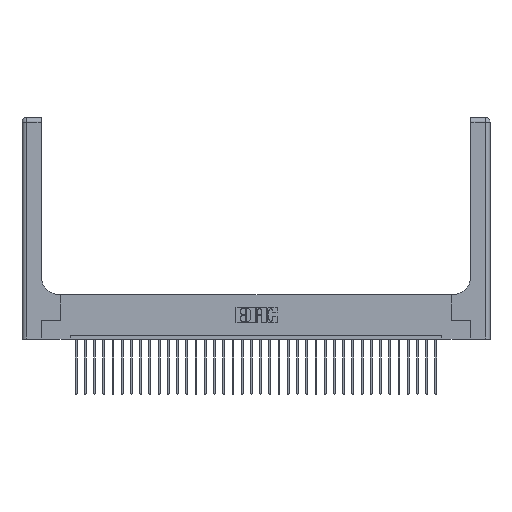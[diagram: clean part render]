
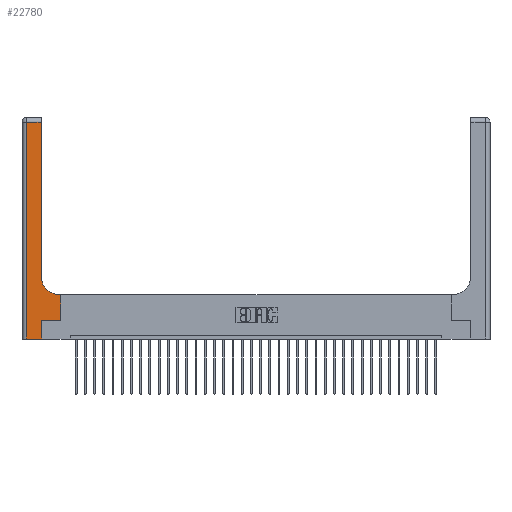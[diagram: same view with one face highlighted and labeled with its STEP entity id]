
A CAD part, top view. The second image highlights one B-rep face of the part: STEP entity #22780.
In plain terms, the highlighted planar face has unit normal (0, 0, 1).
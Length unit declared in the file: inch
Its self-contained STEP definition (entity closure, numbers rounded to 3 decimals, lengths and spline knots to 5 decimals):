
#1024 = CARTESIAN_POINT ( 'NONE',  ( 0.26, 2.94, 0.37 ) ) ;
#1397 = CARTESIAN_POINT ( 'NONE',  ( 0.26, 3., 0.37 ) ) ;
#1685 = CARTESIAN_POINT ( 'NONE',  ( 0., 3., 0.37 ) ) ;
#1891 = DIRECTION ( 'NONE',  ( 0., 0., -1. ) ) ;
#1976 = ORIENTED_EDGE ( 'NONE', *, *, #28139, .T. ) ;
#3897 = DIRECTION ( 'NONE',  ( 0., 1., 0. ) ) ;
#4067 = EDGE_CURVE ( 'NONE', #28895, #26135, #25489, .T. ) ;
#4307 = CARTESIAN_POINT ( 'NONE',  ( 0.06, 3., 0.37 ) ) ;
#4350 = CARTESIAN_POINT ( 'NONE',  ( 0.528, 0.25, 0.37 ) ) ;
#4663 = EDGE_CURVE ( 'NONE', #26135, #20665, #19609, .T. ) ;
#5077 = ORIENTED_EDGE ( 'NONE', *, *, #6929, .T. ) ;
#5150 = VECTOR ( 'NONE', #18084, 39.37008 ) ;
#6020 = ORIENTED_EDGE ( 'NONE', *, *, #16558, .T. ) ;
#6377 = VERTEX_POINT ( 'NONE', #14518 ) ;
#6764 = VECTOR ( 'NONE', #26221, 39.37008 ) ;
#6796 = EDGE_CURVE ( 'NONE', #28186, #12168, #22173, .T. ) ;
#6875 = LINE ( 'NONE', #29794, #18598 ) ;
#6929 = EDGE_CURVE ( 'NONE', #6377, #28895, #21804, .T. ) ;
#8192 = CARTESIAN_POINT ( 'NONE',  ( 0.51, 0.85, 0.37 ) ) ;
#8345 = VERTEX_POINT ( 'NONE', #26158 ) ;
#8560 = EDGE_CURVE ( 'NONE', #29387, #16786, #12880, .T. ) ;
#9217 = ORIENTED_EDGE ( 'NONE', *, *, #4663, .T. ) ;
#9361 = VECTOR ( 'NONE', #21177, 39.37008 ) ;
#9370 = CARTESIAN_POINT ( 'NONE',  ( 0.06, 0., 0.37 ) ) ;
#11215 = CARTESIAN_POINT ( 'NONE',  ( 0.528, 0.6, 0.37 ) ) ;
#11298 = DIRECTION ( 'NONE',  ( 0., -1., 0. ) ) ;
#11910 = FACE_OUTER_BOUND ( 'NONE', #14906, .T. ) ;
#12168 = VERTEX_POINT ( 'NONE', #1024 ) ;
#12880 = LINE ( 'NONE', #4307, #27166 ) ;
#13280 = ORIENTED_EDGE ( 'NONE', *, *, #8560, .T. ) ;
#13945 = CIRCLE ( 'NONE', #25752, 0.25 ) ;
#14185 = DIRECTION ( 'NONE',  ( -1., 0., 0. ) ) ;
#14518 = CARTESIAN_POINT ( 'NONE',  ( 0.265, 0.25, 0.37 ) ) ;
#14860 = ORIENTED_EDGE ( 'NONE', *, *, #6796, .T. ) ;
#14906 = EDGE_LOOP ( 'NONE', ( #14860, #6020, #13280, #19827, #1976, #5077, #29991, #9217, #23270 ) ) ;
#15052 = DIRECTION ( 'NONE',  ( 1., 0., 0. ) ) ;
#15379 = AXIS2_PLACEMENT_3D ( 'NONE', #1685, #1891, #22839 ) ;
#15448 = DIRECTION ( 'NONE',  ( 0., 0., -1. ) ) ;
#15474 = CARTESIAN_POINT ( 'NONE',  ( 0.26, 0.85, 0.37 ) ) ;
#15578 = PLANE ( 'NONE',  #15379 ) ;
#15915 = VECTOR ( 'NONE', #14185, 39.37008 ) ;
#16093 = CARTESIAN_POINT ( 'NONE',  ( 0., 0., 0.37 ) ) ;
#16178 = CARTESIAN_POINT ( 'NONE',  ( 0.528, 0.25, 0.37 ) ) ;
#16558 = EDGE_CURVE ( 'NONE', #12168, #29387, #22740, .T. ) ;
#16786 = VERTEX_POINT ( 'NONE', #9370 ) ;
#18084 = DIRECTION ( 'NONE',  ( -1., 0., 0. ) ) ;
#18189 = CARTESIAN_POINT ( 'NONE',  ( 0.51, 0.6, 0.37 ) ) ;
#18524 = DIRECTION ( 'NONE',  ( 0., 1., 0. ) ) ;
#18598 = VECTOR ( 'NONE', #3897, 39.37008 ) ;
#18666 = EDGE_CURVE ( 'NONE', #20665, #28186, #13945, .T. ) ;
#19609 = LINE ( 'NONE', #27932, #15915 ) ;
#19827 = ORIENTED_EDGE ( 'NONE', *, *, #22883, .T. ) ;
#20665 = VERTEX_POINT ( 'NONE', #18189 ) ;
#21053 = VECTOR ( 'NONE', #27157, 39.37008 ) ;
#21177 = DIRECTION ( 'NONE',  ( 1., 0., 0. ) ) ;
#21280 = CARTESIAN_POINT ( 'NONE',  ( 0.265, 0.25, 0.37 ) ) ;
#21804 = LINE ( 'NONE', #21280, #9361 ) ;
#22173 = LINE ( 'NONE', #1397, #21053 ) ;
#22593 = CARTESIAN_POINT ( 'NONE',  ( 0., 2.94, 0.37 ) ) ;
#22740 = LINE ( 'NONE', #22593, #5150 ) ;
#22780 = ADVANCED_FACE ( 'NONE', ( #11910 ), #15578, .F. ) ;
#22839 = DIRECTION ( 'NONE',  ( -1., 0., 0. ) ) ;
#22883 = EDGE_CURVE ( 'NONE', #16786, #8345, #24342, .T. ) ;
#23270 = ORIENTED_EDGE ( 'NONE', *, *, #18666, .T. ) ;
#24342 = LINE ( 'NONE', #16093, #6764 ) ;
#25489 = LINE ( 'NONE', #16178, #29468 ) ;
#25752 = AXIS2_PLACEMENT_3D ( 'NONE', #8192, #15448, #15052 ) ;
#26135 = VERTEX_POINT ( 'NONE', #11215 ) ;
#26158 = CARTESIAN_POINT ( 'NONE',  ( 0.265, 0., 0.37 ) ) ;
#26221 = DIRECTION ( 'NONE',  ( 1., 0., 0. ) ) ;
#26980 = CARTESIAN_POINT ( 'NONE',  ( 0.06, 2.94, 0.37 ) ) ;
#27157 = DIRECTION ( 'NONE',  ( 0., 1., 0. ) ) ;
#27166 = VECTOR ( 'NONE', #11298, 39.37008 ) ;
#27932 = CARTESIAN_POINT ( 'NONE',  ( 0.26, 0.6, 0.37 ) ) ;
#28139 = EDGE_CURVE ( 'NONE', #8345, #6377, #6875, .T. ) ;
#28186 = VERTEX_POINT ( 'NONE', #15474 ) ;
#28895 = VERTEX_POINT ( 'NONE', #4350 ) ;
#29387 = VERTEX_POINT ( 'NONE', #26980 ) ;
#29468 = VECTOR ( 'NONE', #18524, 39.37008 ) ;
#29794 = CARTESIAN_POINT ( 'NONE',  ( 0.265, 0., 0.37 ) ) ;
#29991 = ORIENTED_EDGE ( 'NONE', *, *, #4067, .T. ) ;
